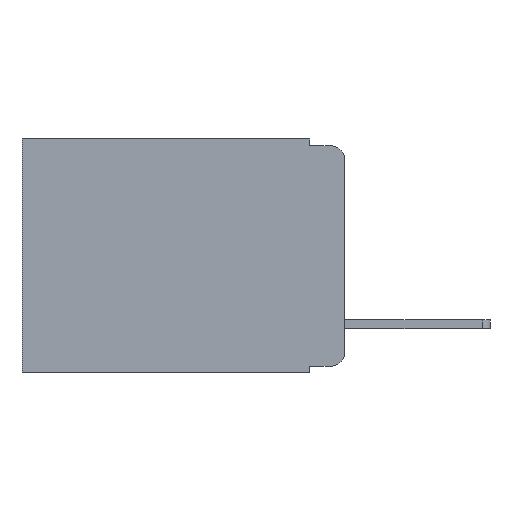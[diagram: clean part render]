
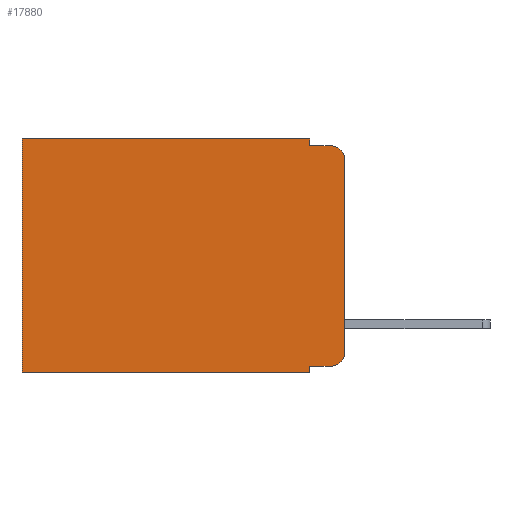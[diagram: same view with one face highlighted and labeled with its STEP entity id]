
A CAD part, left-side view. The second image highlights one B-rep face of the part: STEP entity #17880.
In plain terms, the highlighted planar face has unit normal (-1, 0, 0).
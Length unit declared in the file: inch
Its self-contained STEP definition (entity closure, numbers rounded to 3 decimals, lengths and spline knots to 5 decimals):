
#110 = CARTESIAN_POINT ( 'NONE',  ( 0.298, 0.051, 0. ) ) ;
#289 = VECTOR ( 'NONE', #323, 39.37008 ) ;
#323 = DIRECTION ( 'NONE',  ( 0., -1., 0. ) ) ;
#696 = VECTOR ( 'NONE', #11681, 39.37008 ) ;
#840 = LINE ( 'NONE', #13857, #289 ) ;
#1416 = ORIENTED_EDGE ( 'NONE', *, *, #8350, .T. ) ;
#1529 = CARTESIAN_POINT ( 'NONE',  ( 0.298, 0.051, 0. ) ) ;
#1563 = PLANE ( 'NONE',  #10815 ) ;
#2143 = VERTEX_POINT ( 'NONE', #10945 ) ;
#2306 = VERTEX_POINT ( 'NONE', #15513 ) ;
#2535 = VERTEX_POINT ( 'NONE', #110 ) ;
#2738 = VERTEX_POINT ( 'NONE', #10871 ) ;
#2899 = DIRECTION ( 'NONE',  ( 0., 1., 0. ) ) ;
#3161 = FACE_OUTER_BOUND ( 'NONE', #4857, .T. ) ;
#3285 = DIRECTION ( 'NONE',  ( -1., 0., 0. ) ) ;
#3350 = DIRECTION ( 'NONE',  ( 1., 0., 0. ) ) ;
#3699 = AXIS2_PLACEMENT_3D ( 'NONE', #16809, #3285, #9474 ) ;
#3788 = CARTESIAN_POINT ( 'NONE',  ( 0.298, 0.051, -0.333 ) ) ;
#4337 = CARTESIAN_POINT ( 'NONE',  ( 0.298, 0.02, -0.03 ) ) ;
#4629 = VECTOR ( 'NONE', #18215, 39.37008 ) ;
#4857 = EDGE_LOOP ( 'NONE', ( #13294, #17580, #13797, #18089, #14298, #1416, #6531, #15275, #7048, #15777 ) ) ;
#5032 = EDGE_CURVE ( 'NONE', #15143, #2143, #18721, .T. ) ;
#5070 = CARTESIAN_POINT ( 'NONE',  ( 0.298, 0., 0. ) ) ;
#5296 = CARTESIAN_POINT ( 'NONE',  ( 0.298, 0.02, -0.333 ) ) ;
#5749 = DIRECTION ( 'NONE',  ( 0., 1., 0. ) ) ;
#5839 = VECTOR ( 'NONE', #17354, 39.37008 ) ;
#6007 = DIRECTION ( 'NONE',  ( 0., 0., -1. ) ) ;
#6129 = EDGE_CURVE ( 'NONE', #11984, #15143, #14619, .T. ) ;
#6336 = LINE ( 'NONE', #7334, #10769 ) ;
#6531 = ORIENTED_EDGE ( 'NONE', *, *, #8196, .F. ) ;
#6726 = CARTESIAN_POINT ( 'NONE',  ( 0.298, 0.473, 0. ) ) ;
#6752 = CARTESIAN_POINT ( 'NONE',  ( 0.298, 0.473, 0. ) ) ;
#7048 = ORIENTED_EDGE ( 'NONE', *, *, #6129, .T. ) ;
#7234 = EDGE_CURVE ( 'NONE', #11984, #7786, #6336, .T. ) ;
#7334 = CARTESIAN_POINT ( 'NONE',  ( 0.298, 0.051, 0. ) ) ;
#7626 = LINE ( 'NONE', #5070, #11563 ) ;
#7786 = VERTEX_POINT ( 'NONE', #10313 ) ;
#8186 = AXIS2_PLACEMENT_3D ( 'NONE', #4337, #15855, #6007 ) ;
#8196 = EDGE_CURVE ( 'NONE', #7786, #13177, #12222, .T. ) ;
#8315 = CARTESIAN_POINT ( 'NONE',  ( 0.298, 0., 0. ) ) ;
#8350 = EDGE_CURVE ( 'NONE', #17254, #13177, #9057, .T. ) ;
#8389 = DIRECTION ( 'NONE',  ( 0., 0., -1. ) ) ;
#9057 = LINE ( 'NONE', #6726, #4629 ) ;
#9161 = EDGE_CURVE ( 'NONE', #2535, #17254, #15940, .T. ) ;
#9474 = DIRECTION ( 'NONE',  ( 0., 0., -1. ) ) ;
#9696 = CARTESIAN_POINT ( 'NONE',  ( 0.298, 0., -0.03 ) ) ;
#9999 = CIRCLE ( 'NONE', #8186, 0.02 ) ;
#10313 = CARTESIAN_POINT ( 'NONE',  ( 0.298, 0.051, -0.343 ) ) ;
#10606 = EDGE_CURVE ( 'NONE', #2535, #2738, #13669, .T. ) ;
#10769 = VECTOR ( 'NONE', #13948, 39.37008 ) ;
#10815 = AXIS2_PLACEMENT_3D ( 'NONE', #8315, #3350, #14941 ) ;
#10871 = CARTESIAN_POINT ( 'NONE',  ( 0.298, 0.051, -0.01 ) ) ;
#10945 = CARTESIAN_POINT ( 'NONE',  ( 0.298, 0., -0.313 ) ) ;
#11274 = CARTESIAN_POINT ( 'NONE',  ( 0.298, 0., -0.343 ) ) ;
#11563 = VECTOR ( 'NONE', #8389, 39.37008 ) ;
#11681 = DIRECTION ( 'NONE',  ( 0., 0., -1. ) ) ;
#11984 = VERTEX_POINT ( 'NONE', #13824 ) ;
#12222 = LINE ( 'NONE', #11274, #20288 ) ;
#12831 = EDGE_CURVE ( 'NONE', #2738, #2306, #840, .T. ) ;
#13177 = VERTEX_POINT ( 'NONE', #19468 ) ;
#13294 = ORIENTED_EDGE ( 'NONE', *, *, #17901, .F. ) ;
#13669 = LINE ( 'NONE', #1529, #696 ) ;
#13797 = ORIENTED_EDGE ( 'NONE', *, *, #12831, .F. ) ;
#13824 = CARTESIAN_POINT ( 'NONE',  ( 0.298, 0.051, -0.333 ) ) ;
#13857 = CARTESIAN_POINT ( 'NONE',  ( 0.298, 0.051, -0.01 ) ) ;
#13948 = DIRECTION ( 'NONE',  ( 0., 0., -1. ) ) ;
#14298 = ORIENTED_EDGE ( 'NONE', *, *, #9161, .T. ) ;
#14619 = LINE ( 'NONE', #3788, #5839 ) ;
#14941 = DIRECTION ( 'NONE',  ( 0., 0., -1. ) ) ;
#15143 = VERTEX_POINT ( 'NONE', #5296 ) ;
#15275 = ORIENTED_EDGE ( 'NONE', *, *, #7234, .F. ) ;
#15513 = CARTESIAN_POINT ( 'NONE',  ( 0.298, 0.02, -0.01 ) ) ;
#15777 = ORIENTED_EDGE ( 'NONE', *, *, #5032, .T. ) ;
#15855 = DIRECTION ( 'NONE',  ( -1., 0., 0. ) ) ;
#15940 = LINE ( 'NONE', #17247, #20251 ) ;
#16809 = CARTESIAN_POINT ( 'NONE',  ( 0.298, 0.02, -0.313 ) ) ;
#17247 = CARTESIAN_POINT ( 'NONE',  ( 0.298, 0., 0. ) ) ;
#17254 = VERTEX_POINT ( 'NONE', #6752 ) ;
#17354 = DIRECTION ( 'NONE',  ( 0., -1., 0. ) ) ;
#17580 = ORIENTED_EDGE ( 'NONE', *, *, #20388, .T. ) ;
#17880 = ADVANCED_FACE ( 'NONE', ( #3161 ), #1563, .F. ) ;
#17901 = EDGE_CURVE ( 'NONE', #19302, #2143, #7626, .T. ) ;
#18089 = ORIENTED_EDGE ( 'NONE', *, *, #10606, .F. ) ;
#18215 = DIRECTION ( 'NONE',  ( 0., 0., -1. ) ) ;
#18721 = CIRCLE ( 'NONE', #3699, 0.02 ) ;
#19302 = VERTEX_POINT ( 'NONE', #9696 ) ;
#19468 = CARTESIAN_POINT ( 'NONE',  ( 0.298, 0.473, -0.343 ) ) ;
#20251 = VECTOR ( 'NONE', #5749, 39.37008 ) ;
#20288 = VECTOR ( 'NONE', #2899, 39.37008 ) ;
#20388 = EDGE_CURVE ( 'NONE', #19302, #2306, #9999, .T. ) ;
